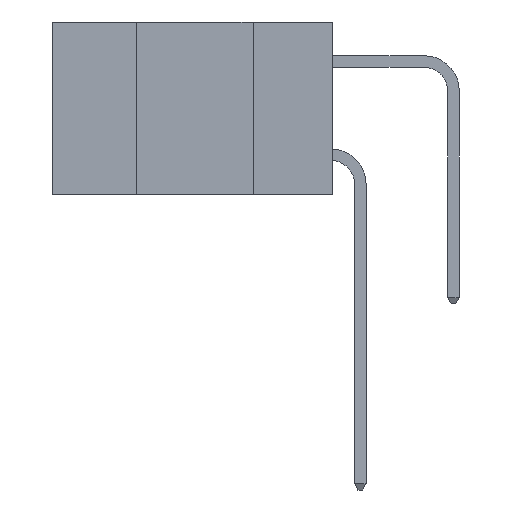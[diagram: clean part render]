
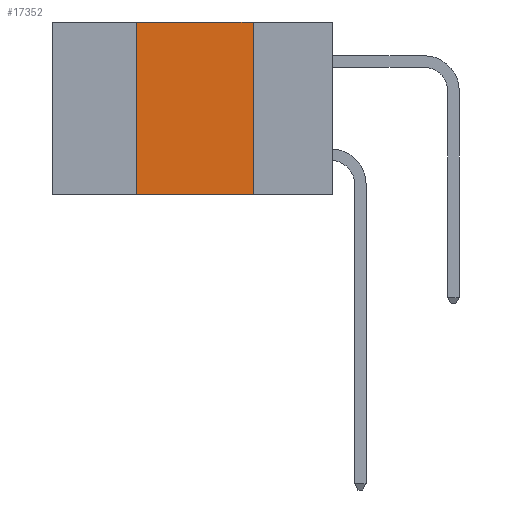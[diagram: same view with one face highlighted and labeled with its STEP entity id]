
A CAD part, left-side view. The second image highlights one B-rep face of the part: STEP entity #17352.
In plain terms, the highlighted planar face has unit normal (-1, 0, 0).
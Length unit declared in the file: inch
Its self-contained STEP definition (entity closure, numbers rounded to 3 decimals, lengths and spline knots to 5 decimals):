
#433 = AXIS2_PLACEMENT_3D ( 'NONE', #11159, #15357, #7044 ) ;
#783 = EDGE_CURVE ( 'NONE', #12989, #15707, #4647, .T. ) ;
#1269 = LINE ( 'NONE', #14809, #15572 ) ;
#1914 = LINE ( 'NONE', #4653, #5169 ) ;
#1932 = EDGE_LOOP ( 'NONE', ( #5855, #7890, #9071, #11132 ) ) ;
#4647 = LINE ( 'NONE', #5336, #11993 ) ;
#4653 = CARTESIAN_POINT ( 'NONE',  ( 0., 0.42, -0.37 ) ) ;
#4675 = VERTEX_POINT ( 'NONE', #9967 ) ;
#5147 = DIRECTION ( 'NONE',  ( 0., -1., 0. ) ) ;
#5169 = VECTOR ( 'NONE', #14333, 39.37008 ) ;
#5336 = CARTESIAN_POINT ( 'NONE',  ( 0., 0.17, -0.37 ) ) ;
#5583 = PLANE ( 'NONE',  #433 ) ;
#5855 = ORIENTED_EDGE ( 'NONE', *, *, #783, .F. ) ;
#7044 = DIRECTION ( 'NONE',  ( 0., 0., -1. ) ) ;
#7890 = ORIENTED_EDGE ( 'NONE', *, *, #17730, .F. ) ;
#8024 = DIRECTION ( 'NONE',  ( 0., -1., 0. ) ) ;
#8240 = FACE_OUTER_BOUND ( 'NONE', #1932, .T. ) ;
#8264 = DIRECTION ( 'NONE',  ( 0., 0., -1. ) ) ;
#8477 = VERTEX_POINT ( 'NONE', #14984 ) ;
#9071 = ORIENTED_EDGE ( 'NONE', *, *, #16881, .F. ) ;
#9967 = CARTESIAN_POINT ( 'NONE',  ( 0., 0.42, -0.37 ) ) ;
#11132 = ORIENTED_EDGE ( 'NONE', *, *, #15985, .T. ) ;
#11159 = CARTESIAN_POINT ( 'NONE',  ( 0., 0.6, 0. ) ) ;
#11993 = VECTOR ( 'NONE', #8264, 39.37008 ) ;
#12131 = VECTOR ( 'NONE', #8024, 39.37008 ) ;
#12989 = VERTEX_POINT ( 'NONE', #17104 ) ;
#14333 = DIRECTION ( 'NONE',  ( 0., 0., 1. ) ) ;
#14809 = CARTESIAN_POINT ( 'NONE',  ( 0., 0.6, 0. ) ) ;
#14984 = CARTESIAN_POINT ( 'NONE',  ( 0., 0.42, 0. ) ) ;
#15357 = DIRECTION ( 'NONE',  ( 1., 0., 0. ) ) ;
#15572 = VECTOR ( 'NONE', #5147, 39.37008 ) ;
#15707 = VERTEX_POINT ( 'NONE', #15785 ) ;
#15785 = CARTESIAN_POINT ( 'NONE',  ( 0., 0.17, -0.37 ) ) ;
#15844 = LINE ( 'NONE', #17625, #12131 ) ;
#15985 = EDGE_CURVE ( 'NONE', #4675, #15707, #15844, .T. ) ;
#16881 = EDGE_CURVE ( 'NONE', #4675, #8477, #1914, .T. ) ;
#17104 = CARTESIAN_POINT ( 'NONE',  ( 0., 0.17, 0. ) ) ;
#17352 = ADVANCED_FACE ( 'NONE', ( #8240 ), #5583, .F. ) ;
#17625 = CARTESIAN_POINT ( 'NONE',  ( 0., 0.6, -0.37 ) ) ;
#17730 = EDGE_CURVE ( 'NONE', #8477, #12989, #1269, .T. ) ;
